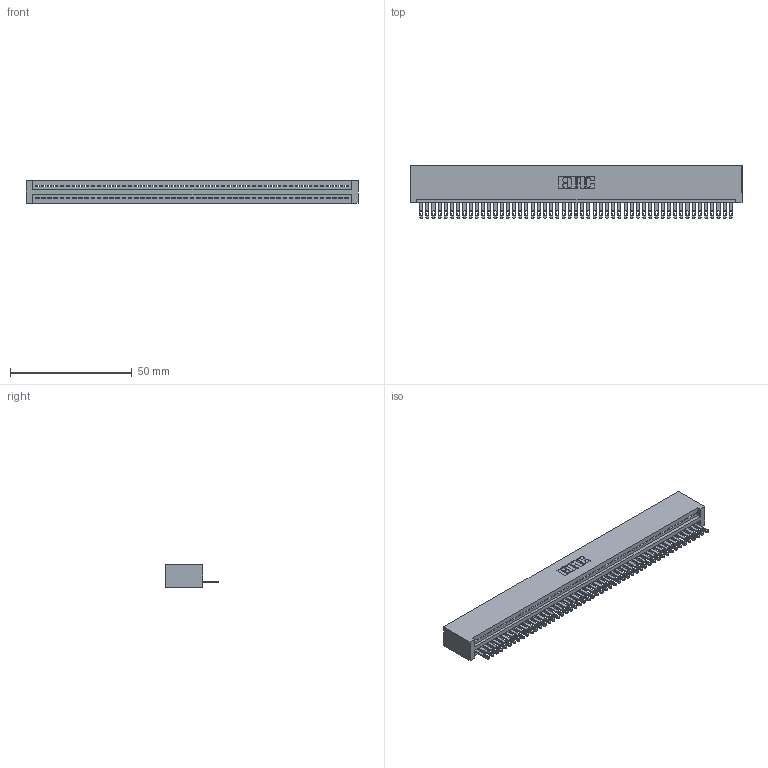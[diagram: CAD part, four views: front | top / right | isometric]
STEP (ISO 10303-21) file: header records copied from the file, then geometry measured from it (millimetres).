
FILE_DESCRIPTION (( 'STEP AP203' ), '1' );
FILE_NAME ('895-051-500-101.STEP', '2020-09-27T09:59:02', ( '' ), ( '' ), 'SwSTEP 2.0', 'SolidWorks 2020', '' );
FILE_SCHEMA (( 'CONFIG_CONTROL_DESIGN' ));
Length unit declared in the file: inch
Products named in the file (3): 895-051-500-101; 345-292-001_345-293-100; 845 Part_No Mounting Lugs
Assembly tree (52 placements, depth 2):
  895-051-500-101
    845 Part_No Mounting Lugs
    345-292-001_345-293-100  x51
Bounding box: 136.14 x 21.51 x 9.4 mm (x, y, z)
Volume: 13620.7 mm3; surface area: 18527.7 mm2
Topology: 52 solids, 52 shells, 2872 faces, 8885 edges, 5922 vertices
Faces by surface type: plane 1810, cylinder 1062
Entity records: 36825 total; most frequent: CARTESIAN_POINT 6385, ORIENTED_EDGE 6370, DIRECTION 5559, EDGE_CURVE 3185, VECTOR 2853, LINE 2853, VERTEX_POINT 2122, AXIS2_PLACEMENT_3D 1353
